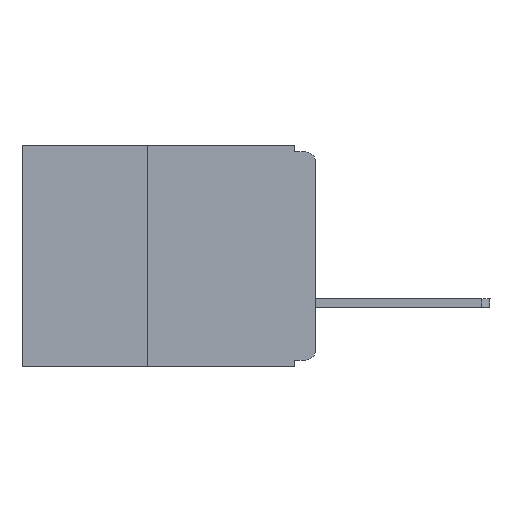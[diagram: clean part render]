
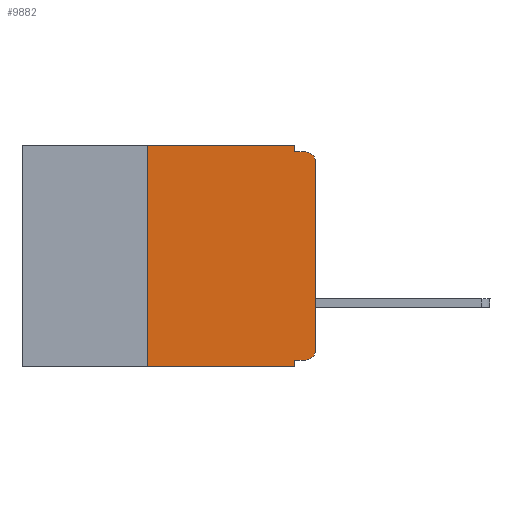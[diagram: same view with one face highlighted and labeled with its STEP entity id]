
A CAD part, left-side view. The second image highlights one B-rep face of the part: STEP entity #9882.
In plain terms, the highlighted planar face has unit normal (-1, 0, 0).
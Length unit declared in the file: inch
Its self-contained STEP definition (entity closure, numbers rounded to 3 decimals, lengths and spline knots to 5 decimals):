
#249 = VERTEX_POINT ( 'NONE', #8141 ) ;
#266 = ORIENTED_EDGE ( 'NONE', *, *, #2719, .T. ) ;
#280 = DIRECTION ( 'NONE',  ( 0., 0., -1. ) ) ;
#662 = VERTEX_POINT ( 'NONE', #5138 ) ;
#682 = ORIENTED_EDGE ( 'NONE', *, *, #4987, .F. ) ;
#902 = VERTEX_POINT ( 'NONE', #8206 ) ;
#932 = EDGE_CURVE ( 'NONE', #662, #1057, #2909, .T. ) ;
#1033 = EDGE_CURVE ( 'NONE', #662, #2908, #5474, .T. ) ;
#1057 = VERTEX_POINT ( 'NONE', #4988 ) ;
#1109 = CARTESIAN_POINT ( 'NONE',  ( 0., 0.031, -0.33 ) ) ;
#1182 = EDGE_CURVE ( 'NONE', #902, #9157, #8211, .T. ) ;
#1222 = DIRECTION ( 'NONE',  ( 0., -1., 0. ) ) ;
#1272 = EDGE_CURVE ( 'NONE', #9157, #249, #7552, .T. ) ;
#1287 = VECTOR ( 'NONE', #280, 39.37008 ) ;
#1300 = VECTOR ( 'NONE', #2979, 39.37008 ) ;
#1374 = CARTESIAN_POINT ( 'NONE',  ( 0., 0., -0.32 ) ) ;
#1484 = ORIENTED_EDGE ( 'NONE', *, *, #6426, .F. ) ;
#1808 = CARTESIAN_POINT ( 'NONE',  ( 0., 0.031, -0.33 ) ) ;
#2037 = AXIS2_PLACEMENT_3D ( 'NONE', #3749, #2941, #9834 ) ;
#2169 = VERTEX_POINT ( 'NONE', #8896 ) ;
#2286 = DIRECTION ( 'NONE',  ( 0., 0., -1. ) ) ;
#2511 = AXIS2_PLACEMENT_3D ( 'NONE', #4799, #5757, #5720 ) ;
#2574 = VERTEX_POINT ( 'NONE', #1808 ) ;
#2703 = CARTESIAN_POINT ( 'NONE',  ( 0., 0., 0. ) ) ;
#2719 = EDGE_CURVE ( 'NONE', #7698, #249, #3275, .T. ) ;
#2871 = LINE ( 'NONE', #1109, #4905 ) ;
#2898 = VECTOR ( 'NONE', #1222, 39.37008 ) ;
#2902 = CARTESIAN_POINT ( 'NONE',  ( 0., 0., -0.01 ) ) ;
#2908 = VERTEX_POINT ( 'NONE', #10277 ) ;
#2909 = LINE ( 'NONE', #1374, #1300 ) ;
#2915 = VECTOR ( 'NONE', #9891, 39.37008 ) ;
#2941 = DIRECTION ( 'NONE',  ( -1., 0., 0. ) ) ;
#2979 = DIRECTION ( 'NONE',  ( 0., 1., 0. ) ) ;
#3275 = CIRCLE ( 'NONE', #2037, 0.015 ) ;
#3323 = LINE ( 'NONE', #10636, #2915 ) ;
#3331 = VECTOR ( 'NONE', #6063, 39.37008 ) ;
#3603 = LINE ( 'NONE', #11234, #3331 ) ;
#3749 = CARTESIAN_POINT ( 'NONE',  ( 0., 0.015, -0.025 ) ) ;
#3757 = ORIENTED_EDGE ( 'NONE', *, *, #1033, .T. ) ;
#3785 = FACE_OUTER_BOUND ( 'NONE', #10422, .T. ) ;
#4200 = DIRECTION ( 'NONE',  ( -1., 0., 0. ) ) ;
#4256 = VECTOR ( 'NONE', #6631, 39.37008 ) ;
#4277 = ORIENTED_EDGE ( 'NONE', *, *, #1182, .F. ) ;
#4509 = LINE ( 'NONE', #7106, #5190 ) ;
#4626 = ORIENTED_EDGE ( 'NONE', *, *, #10934, .T. ) ;
#4799 = CARTESIAN_POINT ( 'NONE',  ( 0., 0.437, 0. ) ) ;
#4836 = PLANE ( 'NONE',  #2511 ) ;
#4905 = VECTOR ( 'NONE', #7228, 39.37008 ) ;
#4987 = EDGE_CURVE ( 'NONE', #9024, #902, #3603, .T. ) ;
#4988 = CARTESIAN_POINT ( 'NONE',  ( 0., 0.031, -0.32 ) ) ;
#5138 = CARTESIAN_POINT ( 'NONE',  ( 0., 0.015, -0.32 ) ) ;
#5190 = VECTOR ( 'NONE', #5255, 39.37008 ) ;
#5255 = DIRECTION ( 'NONE',  ( 0., 0., 1. ) ) ;
#5397 = CARTESIAN_POINT ( 'NONE',  ( 0., 0.031, 0. ) ) ;
#5442 = CARTESIAN_POINT ( 'NONE',  ( 0., 0., -0.025 ) ) ;
#5474 = CIRCLE ( 'NONE', #9958, 0.015 ) ;
#5720 = DIRECTION ( 'NONE',  ( 0., 0., -1. ) ) ;
#5757 = DIRECTION ( 'NONE',  ( 1., 0., 0. ) ) ;
#5987 = ORIENTED_EDGE ( 'NONE', *, *, #932, .F. ) ;
#6063 = DIRECTION ( 'NONE',  ( 0., -1., 0. ) ) ;
#6067 = EDGE_CURVE ( 'NONE', #2908, #7698, #8887, .T. ) ;
#6426 = EDGE_CURVE ( 'NONE', #2169, #9024, #4509, .T. ) ;
#6497 = ORIENTED_EDGE ( 'NONE', *, *, #6067, .T. ) ;
#6631 = DIRECTION ( 'NONE',  ( 0., 0., 1. ) ) ;
#7106 = CARTESIAN_POINT ( 'NONE',  ( 0., 0.25, -0.33 ) ) ;
#7228 = DIRECTION ( 'NONE',  ( 0., 0., -1. ) ) ;
#7535 = CARTESIAN_POINT ( 'NONE',  ( 0., 0.015, -0.305 ) ) ;
#7552 = LINE ( 'NONE', #2902, #2898 ) ;
#7625 = EDGE_CURVE ( 'NONE', #1057, #2574, #2871, .T. ) ;
#7698 = VERTEX_POINT ( 'NONE', #5442 ) ;
#8141 = CARTESIAN_POINT ( 'NONE',  ( 0., 0.015, -0.01 ) ) ;
#8206 = CARTESIAN_POINT ( 'NONE',  ( 0., 0.031, 0. ) ) ;
#8211 = LINE ( 'NONE', #5397, #1287 ) ;
#8552 = CARTESIAN_POINT ( 'NONE',  ( 0., 0.031, -0.01 ) ) ;
#8585 = ORIENTED_EDGE ( 'NONE', *, *, #7625, .F. ) ;
#8887 = LINE ( 'NONE', #2703, #4256 ) ;
#8896 = CARTESIAN_POINT ( 'NONE',  ( 0., 0.25, -0.33 ) ) ;
#9024 = VERTEX_POINT ( 'NONE', #10896 ) ;
#9157 = VERTEX_POINT ( 'NONE', #8552 ) ;
#9834 = DIRECTION ( 'NONE',  ( 0., 0., -1. ) ) ;
#9882 = ADVANCED_FACE ( 'NONE', ( #3785 ), #4836, .F. ) ;
#9891 = DIRECTION ( 'NONE',  ( 0., -1., 0. ) ) ;
#9958 = AXIS2_PLACEMENT_3D ( 'NONE', #7535, #4200, #2286 ) ;
#10277 = CARTESIAN_POINT ( 'NONE',  ( 0., 0., -0.305 ) ) ;
#10422 = EDGE_LOOP ( 'NONE', ( #6497, #266, #11064, #4277, #682, #1484, #4626, #8585, #5987, #3757 ) ) ;
#10636 = CARTESIAN_POINT ( 'NONE',  ( 0., 0.437, -0.33 ) ) ;
#10896 = CARTESIAN_POINT ( 'NONE',  ( 0., 0.25, 0. ) ) ;
#10934 = EDGE_CURVE ( 'NONE', #2169, #2574, #3323, .T. ) ;
#11064 = ORIENTED_EDGE ( 'NONE', *, *, #1272, .F. ) ;
#11234 = CARTESIAN_POINT ( 'NONE',  ( 0., 0.437, 0. ) ) ;
